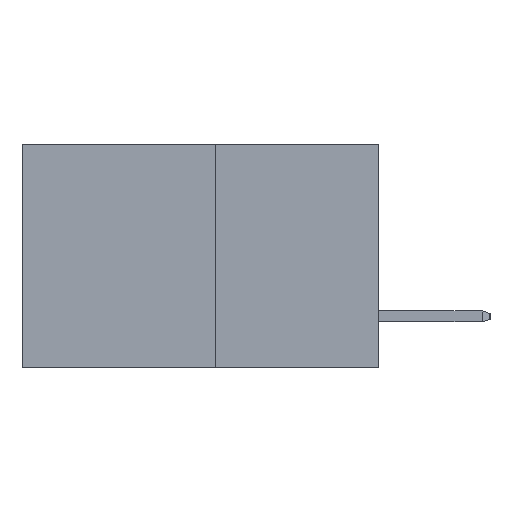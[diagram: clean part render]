
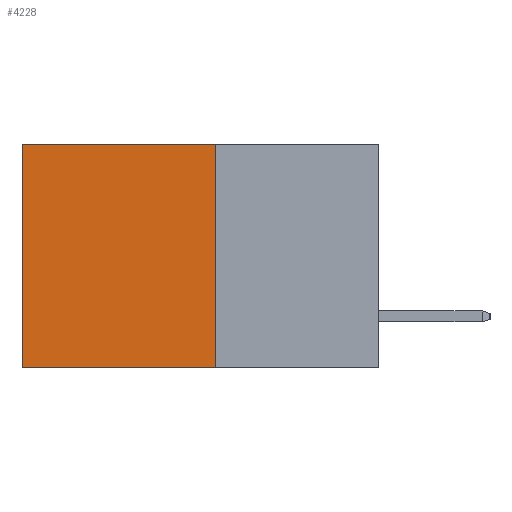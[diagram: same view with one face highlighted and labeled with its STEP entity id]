
A CAD part, left-side view. The second image highlights one B-rep face of the part: STEP entity #4228.
In plain terms, the highlighted planar face has unit normal (-1, 0, 0).
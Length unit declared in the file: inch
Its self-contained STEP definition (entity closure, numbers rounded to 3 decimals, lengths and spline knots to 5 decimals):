
#1221 = EDGE_LOOP ( 'NONE', ( #11615, #6932, #2113, #9798 ) ) ;
#1814 = CARTESIAN_POINT ( 'NONE',  ( 0.277, 0.27, -0.37 ) ) ;
#2054 = VECTOR ( 'NONE', #4344, 39.37008 ) ;
#2113 = ORIENTED_EDGE ( 'NONE', *, *, #20717, .F. ) ;
#2758 = VERTEX_POINT ( 'NONE', #6283 ) ;
#3956 = DIRECTION ( 'NONE',  ( 0., 0., -1. ) ) ;
#4214 = DIRECTION ( 'NONE',  ( 0., 0., -1. ) ) ;
#4228 = ADVANCED_FACE ( 'NONE', ( #7438 ), #4432, .F. ) ;
#4246 = DIRECTION ( 'NONE',  ( 1., 0., 0. ) ) ;
#4328 = CARTESIAN_POINT ( 'NONE',  ( 0.277, 0.27, -0.37 ) ) ;
#4344 = DIRECTION ( 'NONE',  ( 0., 1., 0. ) ) ;
#4432 = PLANE ( 'NONE',  #19031 ) ;
#5141 = CARTESIAN_POINT ( 'NONE',  ( 0.277, 0.27, 0. ) ) ;
#5965 = LINE ( 'NONE', #9428, #21508 ) ;
#6283 = CARTESIAN_POINT ( 'NONE',  ( 0.277, 0.59, 0. ) ) ;
#6519 = EDGE_CURVE ( 'NONE', #2758, #23882, #5965, .T. ) ;
#6932 = ORIENTED_EDGE ( 'NONE', *, *, #10380, .F. ) ;
#7438 = FACE_OUTER_BOUND ( 'NONE', #1221, .T. ) ;
#7710 = LINE ( 'NONE', #16779, #2054 ) ;
#8793 = CARTESIAN_POINT ( 'NONE',  ( 0.277, 0.27, -0.37 ) ) ;
#9428 = CARTESIAN_POINT ( 'NONE',  ( 0.277, 0.59, -0.37 ) ) ;
#9798 = ORIENTED_EDGE ( 'NONE', *, *, #15947, .T. ) ;
#10380 = EDGE_CURVE ( 'NONE', #24358, #23882, #12185, .T. ) ;
#10879 = DIRECTION ( 'NONE',  ( 0., 1., 0. ) ) ;
#10889 = VECTOR ( 'NONE', #10879, 39.37008 ) ;
#11615 = ORIENTED_EDGE ( 'NONE', *, *, #6519, .T. ) ;
#11653 = VERTEX_POINT ( 'NONE', #5141 ) ;
#12185 = LINE ( 'NONE', #8793, #10889 ) ;
#13508 = CARTESIAN_POINT ( 'NONE',  ( 0.277, 0.27, -0.37 ) ) ;
#15947 = EDGE_CURVE ( 'NONE', #11653, #2758, #7710, .T. ) ;
#16779 = CARTESIAN_POINT ( 'NONE',  ( 0.277, 0.27, 0. ) ) ;
#19031 = AXIS2_PLACEMENT_3D ( 'NONE', #4328, #4246, #4214 ) ;
#20717 = EDGE_CURVE ( 'NONE', #11653, #24358, #21621, .T. ) ;
#21015 = VECTOR ( 'NONE', #3956, 39.37008 ) ;
#21508 = VECTOR ( 'NONE', #23388, 39.37008 ) ;
#21621 = LINE ( 'NONE', #1814, #21015 ) ;
#22045 = CARTESIAN_POINT ( 'NONE',  ( 0.277, 0.59, -0.37 ) ) ;
#23388 = DIRECTION ( 'NONE',  ( 0., 0., -1. ) ) ;
#23882 = VERTEX_POINT ( 'NONE', #22045 ) ;
#24358 = VERTEX_POINT ( 'NONE', #13508 ) ;
